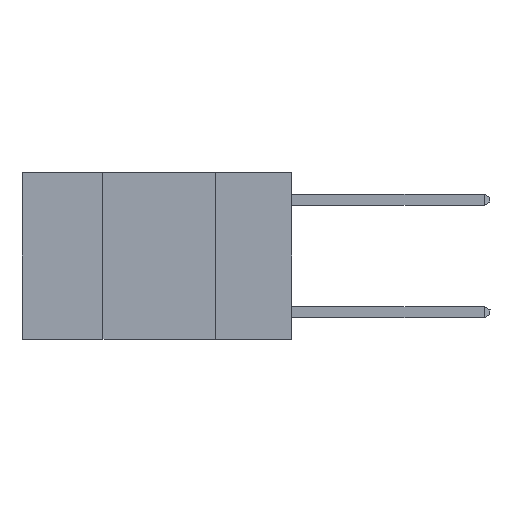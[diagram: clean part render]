
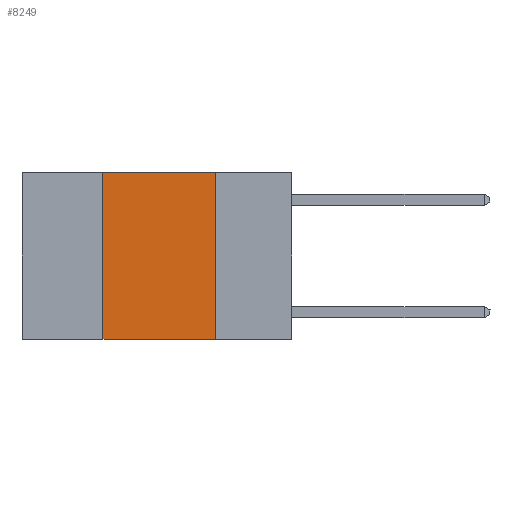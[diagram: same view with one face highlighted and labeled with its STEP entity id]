
A CAD part, left-side view. The second image highlights one B-rep face of the part: STEP entity #8249.
In plain terms, the highlighted planar face has unit normal (-1, 0, 0).
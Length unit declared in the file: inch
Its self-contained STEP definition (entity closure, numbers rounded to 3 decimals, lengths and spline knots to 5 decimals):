
#206 = VECTOR ( 'NONE', #1847, 39.37008 ) ;
#765 = DIRECTION ( 'NONE',  ( 1., 0., 0. ) ) ;
#1068 = ORIENTED_EDGE ( 'NONE', *, *, #2529, .F. ) ;
#1428 = VECTOR ( 'NONE', #2621, 39.37008 ) ;
#1648 = CARTESIAN_POINT ( 'NONE',  ( 0., 0.42, 0. ) ) ;
#1667 = ORIENTED_EDGE ( 'NONE', *, *, #11520, .T. ) ;
#1847 = DIRECTION ( 'NONE',  ( 0., -1., 0. ) ) ;
#2529 = EDGE_CURVE ( 'NONE', #12361, #7694, #8926, .T. ) ;
#2621 = DIRECTION ( 'NONE',  ( 0., 0., -1. ) ) ;
#2796 = LINE ( 'NONE', #8675, #206 ) ;
#3159 = LINE ( 'NONE', #10964, #8650 ) ;
#3617 = CARTESIAN_POINT ( 'NONE',  ( 0., 0.17, 0. ) ) ;
#3871 = EDGE_CURVE ( 'NONE', #11975, #9695, #6603, .T. ) ;
#3872 = CARTESIAN_POINT ( 'NONE',  ( 0., 0.42, 0. ) ) ;
#3874 = FACE_OUTER_BOUND ( 'NONE', #8897, .T. ) ;
#4008 = EDGE_CURVE ( 'NONE', #7694, #11975, #2796, .T. ) ;
#4310 = AXIS2_PLACEMENT_3D ( 'NONE', #4605, #765, #7559 ) ;
#4605 = CARTESIAN_POINT ( 'NONE',  ( 0., 0.6, 0. ) ) ;
#5192 = DIRECTION ( 'NONE',  ( 0., -1., 0. ) ) ;
#6334 = VECTOR ( 'NONE', #9776, 39.37008 ) ;
#6603 = LINE ( 'NONE', #3617, #1428 ) ;
#6784 = CARTESIAN_POINT ( 'NONE',  ( 0., 0.17, 0. ) ) ;
#7559 = DIRECTION ( 'NONE',  ( 0., 0., -1. ) ) ;
#7694 = VERTEX_POINT ( 'NONE', #3872 ) ;
#8105 = CARTESIAN_POINT ( 'NONE',  ( 0., 0.17, -0.37 ) ) ;
#8224 = ORIENTED_EDGE ( 'NONE', *, *, #3871, .F. ) ;
#8249 = ADVANCED_FACE ( 'NONE', ( #3874 ), #12386, .F. ) ;
#8650 = VECTOR ( 'NONE', #5192, 39.37008 ) ;
#8675 = CARTESIAN_POINT ( 'NONE',  ( 0., 0.6, 0. ) ) ;
#8897 = EDGE_LOOP ( 'NONE', ( #8224, #10774, #1068, #1667 ) ) ;
#8926 = LINE ( 'NONE', #1648, #6334 ) ;
#9695 = VERTEX_POINT ( 'NONE', #8105 ) ;
#9776 = DIRECTION ( 'NONE',  ( 0., 0., 1. ) ) ;
#10774 = ORIENTED_EDGE ( 'NONE', *, *, #4008, .F. ) ;
#10964 = CARTESIAN_POINT ( 'NONE',  ( 0., 0.6, -0.37 ) ) ;
#11520 = EDGE_CURVE ( 'NONE', #12361, #9695, #3159, .T. ) ;
#11975 = VERTEX_POINT ( 'NONE', #6784 ) ;
#12166 = CARTESIAN_POINT ( 'NONE',  ( 0., 0.42, -0.37 ) ) ;
#12361 = VERTEX_POINT ( 'NONE', #12166 ) ;
#12386 = PLANE ( 'NONE',  #4310 ) ;
